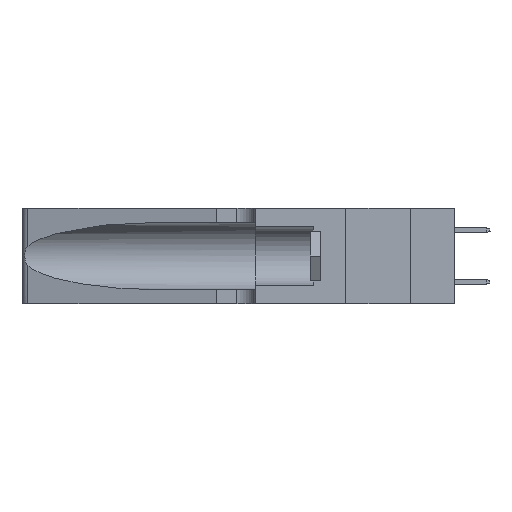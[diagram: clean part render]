
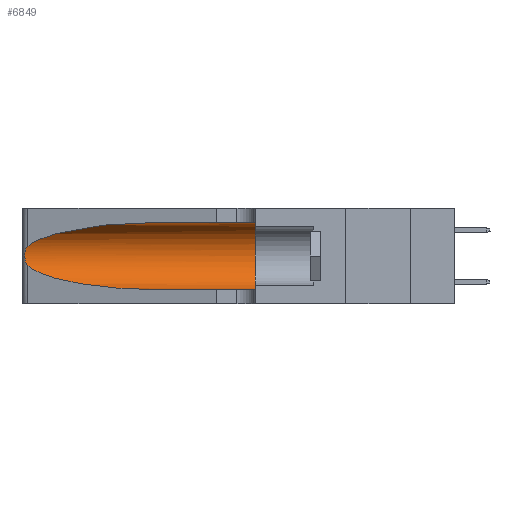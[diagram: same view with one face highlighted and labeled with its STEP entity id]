
A CAD part, left-side view. The second image highlights one B-rep face of the part: STEP entity #6849.
In plain terms, the highlighted cylindrical face has radius 3.308 mm (diameter 6.617 mm), a partial arc.
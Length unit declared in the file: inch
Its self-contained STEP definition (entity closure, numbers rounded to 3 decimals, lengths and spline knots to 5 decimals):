
#410 = CARTESIAN_POINT ( 'NONE',  ( 0.25487, 1.22718, 0.14631 ) ) ;
#613 = CARTESIAN_POINT ( 'NONE',  ( 0.2373, 1.15595, 0.08982 ) ) ;
#914 = CARTESIAN_POINT ( 'NONE',  ( 0.25555, 1.22993, 0.14849 ) ) ;
#1017 = EDGE_CURVE ( 'NONE', #12994, #7404, #23982, .T. ) ;
#1519 = EDGE_CURVE ( 'NONE', #4746, #7404, #27494, .T. ) ;
#2072 = CARTESIAN_POINT ( 'NONE',  ( 0.1305, 1.61858, 0.31525 ) ) ;
#3374 = CARTESIAN_POINT ( 'NONE',  ( 0.26017, 1.23833, 0.17102 ) ) ;
#3464 = CARTESIAN_POINT ( 'NONE',  ( 0.25487, 1.22718, 0.22369 ) ) ;
#3480 = DIRECTION ( 'NONE',  ( 0., -1., 0. ) ) ;
#3847 = CARTESIAN_POINT ( 'NONE',  ( 0.1305, 0.72297, 0.31525 ) ) ;
#4033 = EDGE_CURVE ( 'NONE', #24220, #4746, #14211, .T. ) ;
#4746 = VERTEX_POINT ( 'NONE', #31512 ) ;
#5758 = DIRECTION ( 'NONE',  ( 0., 0., -1. ) ) ;
#6210 = CARTESIAN_POINT ( 'NONE',  ( 0.25487, 1.22718, 0.22369 ) ) ;
#6389 = CARTESIAN_POINT ( 'NONE',  ( 0.25555, 1.22994, 0.2215 ) ) ;
#6587 = CARTESIAN_POINT ( 'NONE',  ( 0.26075, 1.23896, 0.19203 ) ) ;
#6849 = ADVANCED_FACE ( 'NONE', ( #26329 ), #17819, .F. ) ;
#7404 = VERTEX_POINT ( 'NONE', #21295 ) ;
#8910 = CARTESIAN_POINT ( 'NONE',  ( 0.1305, 0.72297, 0.05475 ) ) ;
#8926 =( BOUNDED_CURVE ( )  B_SPLINE_CURVE ( 3, ( #3847, #15345, #23662, #3464 ),
 .UNSPECIFIED., .F., .T. ) 
 B_SPLINE_CURVE_WITH_KNOTS ( ( 4, 4 ),
 ( 1.5708, 2.84003 ),
 .UNSPECIFIED. ) 
 CURVE ( )  GEOMETRIC_REPRESENTATION_ITEM ( )  RATIONAL_B_SPLINE_CURVE ( ( 1., 0.87, 0.87, 1. ) ) 
 REPRESENTATION_ITEM ( '' )  );
#10139 = EDGE_CURVE ( 'NONE', #23956, #11674, #8926, .T. ) ;
#10257 = ORIENTED_EDGE ( 'NONE', *, *, #4033, .T. ) ;
#10450 = EDGE_LOOP ( 'NONE', ( #20445, #19070, #10257, #17597, #32887, #18436 ) ) ;
#11674 = VERTEX_POINT ( 'NONE', #18075 ) ;
#12994 = VERTEX_POINT ( 'NONE', #21128 ) ;
#13752 = CARTESIAN_POINT ( 'NONE',  ( 0.1305, 0.35, 0.185 ) ) ;
#13796 = AXIS2_PLACEMENT_3D ( 'NONE', #29373, #3480, #5758 ) ;
#13903 = CARTESIAN_POINT ( 'NONE',  ( 0.1305, 1.61858, 0.05475 ) ) ;
#14211 =( BOUNDED_CURVE ( )  B_SPLINE_CURVE ( 3, ( #410, #613, #14943, #8910 ),
 .UNSPECIFIED., .F., .T. ) 
 B_SPLINE_CURVE_WITH_KNOTS ( ( 4, 4 ),
 ( 3.44316, 4.71239 ),
 .UNSPECIFIED. ) 
 CURVE ( )  GEOMETRIC_REPRESENTATION_ITEM ( )  RATIONAL_B_SPLINE_CURVE ( ( 1., 0.87, 0.87, 1. ) ) 
 REPRESENTATION_ITEM ( '' )  );
#14343 = EDGE_CURVE ( 'NONE', #23956, #12994, #22247, .T. ) ;
#14885 = CARTESIAN_POINT ( 'NONE',  ( 0.25639, 1.23186, 0.15144 ) ) ;
#14943 = CARTESIAN_POINT ( 'NONE',  ( 0.18966, 0.96281, 0.05475 ) ) ;
#15345 = CARTESIAN_POINT ( 'NONE',  ( 0.18966, 0.96281, 0.31525 ) ) ;
#15547 = AXIS2_PLACEMENT_3D ( 'NONE', #13752, #27742, #22415 ) ;
#16118 = CARTESIAN_POINT ( 'NONE',  ( 0.25854, 1.2359, 0.20912 ) ) ;
#17597 = ORIENTED_EDGE ( 'NONE', *, *, #1519, .T. ) ;
#17819 = CYLINDRICAL_SURFACE ( 'NONE', #13796, 0.13025 ) ;
#18075 = CARTESIAN_POINT ( 'NONE',  ( 0.25487, 1.22718, 0.22369 ) ) ;
#18436 = ORIENTED_EDGE ( 'NONE', *, *, #14343, .F. ) ;
#18989 = B_SPLINE_CURVE_WITH_KNOTS ( 'NONE', 3,
 ( #6210, #6389, #35461, #29461, #16118, #29265, #6587, #26620, #3374, #23926, #27664, #14885, #914, #32461 ),
 .UNSPECIFIED., .F., .F.,
 ( 4, 2, 2, 2, 2, 2, 4 ),
 ( 0., 0.00027, 0.00053, 0.00107, 0.0016, 0.00187, 0.00214 ),
 .UNSPECIFIED. ) ;
#19070 = ORIENTED_EDGE ( 'NONE', *, *, #20463, .T. ) ;
#20445 = ORIENTED_EDGE ( 'NONE', *, *, #10139, .T. ) ;
#20463 = EDGE_CURVE ( 'NONE', #11674, #24220, #18989, .T. ) ;
#20784 = VECTOR ( 'NONE', #22053, 39.37008 ) ;
#21128 = CARTESIAN_POINT ( 'NONE',  ( 0.1305, 0.35, 0.31525 ) ) ;
#21295 = CARTESIAN_POINT ( 'NONE',  ( 0.1305, 0.35, 0.05475 ) ) ;
#22053 = DIRECTION ( 'NONE',  ( 0., -1., 0. ) ) ;
#22247 = LINE ( 'NONE', #2072, #20784 ) ;
#22415 = DIRECTION ( 'NONE',  ( 0., 0., 1. ) ) ;
#23662 = CARTESIAN_POINT ( 'NONE',  ( 0.2373, 1.15595, 0.28018 ) ) ;
#23926 = CARTESIAN_POINT ( 'NONE',  ( 0.25856, 1.23593, 0.16098 ) ) ;
#23956 = VERTEX_POINT ( 'NONE', #36090 ) ;
#23982 = CIRCLE ( 'NONE', #15547, 0.13025 ) ;
#24220 = VERTEX_POINT ( 'NONE', #28365 ) ;
#25438 = DIRECTION ( 'NONE',  ( 0., -1., 0. ) ) ;
#26329 = FACE_OUTER_BOUND ( 'NONE', #10450, .T. ) ;
#26620 = CARTESIAN_POINT ( 'NONE',  ( 0.26075, 1.23896, 0.178 ) ) ;
#27494 = LINE ( 'NONE', #13903, #36710 ) ;
#27664 = CARTESIAN_POINT ( 'NONE',  ( 0.25789, 1.23486, 0.15765 ) ) ;
#27742 = DIRECTION ( 'NONE',  ( 0., 1., 0. ) ) ;
#28365 = CARTESIAN_POINT ( 'NONE',  ( 0.25487, 1.22718, 0.14631 ) ) ;
#29265 = CARTESIAN_POINT ( 'NONE',  ( 0.26018, 1.23835, 0.19895 ) ) ;
#29373 = CARTESIAN_POINT ( 'NONE',  ( 0.1305, 1.61858, 0.185 ) ) ;
#29461 = CARTESIAN_POINT ( 'NONE',  ( 0.25787, 1.23484, 0.2124 ) ) ;
#31512 = CARTESIAN_POINT ( 'NONE',  ( 0.1305, 0.72297, 0.05475 ) ) ;
#32461 = CARTESIAN_POINT ( 'NONE',  ( 0.25487, 1.22718, 0.14631 ) ) ;
#32887 = ORIENTED_EDGE ( 'NONE', *, *, #1017, .F. ) ;
#35461 = CARTESIAN_POINT ( 'NONE',  ( 0.25639, 1.23184, 0.21858 ) ) ;
#36090 = CARTESIAN_POINT ( 'NONE',  ( 0.1305, 0.72297, 0.31525 ) ) ;
#36710 = VECTOR ( 'NONE', #25438, 39.37008 ) ;
